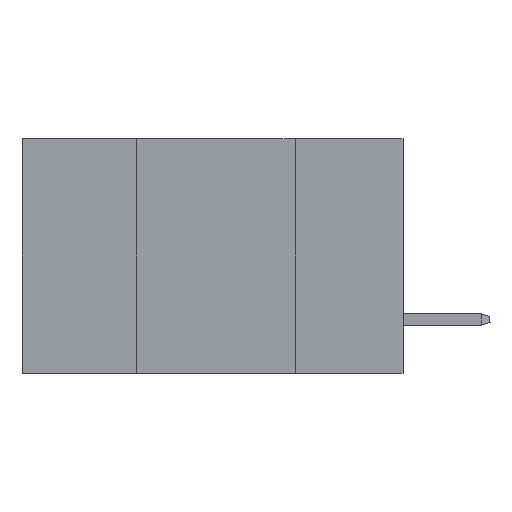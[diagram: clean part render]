
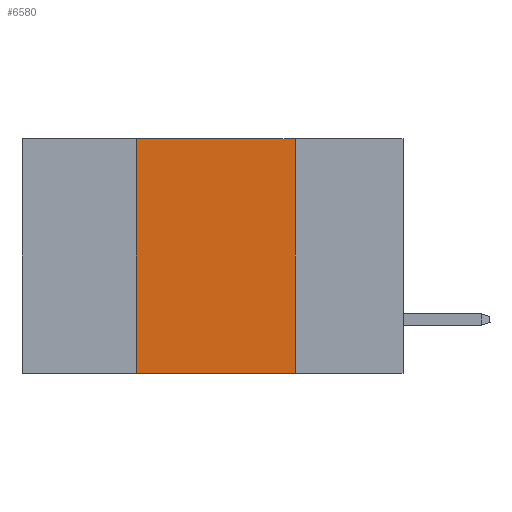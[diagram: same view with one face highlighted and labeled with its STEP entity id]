
A CAD part, left-side view. The second image highlights one B-rep face of the part: STEP entity #6580.
In plain terms, the highlighted planar face has unit normal (-1, 0, 0).
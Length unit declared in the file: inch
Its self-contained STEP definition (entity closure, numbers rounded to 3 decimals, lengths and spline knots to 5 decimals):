
#462 = ORIENTED_EDGE ( 'NONE', *, *, #1246, .F. ) ;
#648 = PLANE ( 'NONE',  #18231 ) ;
#1246 = EDGE_CURVE ( 'NONE', #4660, #2395, #1484, .T. ) ;
#1484 = LINE ( 'NONE', #4633, #2596 ) ;
#2219 = ORIENTED_EDGE ( 'NONE', *, *, #6779, .F. ) ;
#2395 = VERTEX_POINT ( 'NONE', #5164 ) ;
#2596 = VECTOR ( 'NONE', #7207, 39.37008 ) ;
#3591 = DIRECTION ( 'NONE',  ( 1., 0., 0. ) ) ;
#4169 = VERTEX_POINT ( 'NONE', #14268 ) ;
#4259 = DIRECTION ( 'NONE',  ( 0., 0., 1. ) ) ;
#4633 = CARTESIAN_POINT ( 'NONE',  ( 0., 0.6, 0. ) ) ;
#4660 = VERTEX_POINT ( 'NONE', #18342 ) ;
#5164 = CARTESIAN_POINT ( 'NONE',  ( 0., 0.17, 0. ) ) ;
#5970 = CARTESIAN_POINT ( 'NONE',  ( 0., 0.42, 0. ) ) ;
#6441 = CARTESIAN_POINT ( 'NONE',  ( 0., 0.6, 0. ) ) ;
#6580 = ADVANCED_FACE ( 'NONE', ( #13741 ), #648, .F. ) ;
#6779 = EDGE_CURVE ( 'NONE', #4169, #4660, #9993, .T. ) ;
#7207 = DIRECTION ( 'NONE',  ( 0., -1., 0. ) ) ;
#7555 = EDGE_LOOP ( 'NONE', ( #17619, #462, #2219, #8541 ) ) ;
#8541 = ORIENTED_EDGE ( 'NONE', *, *, #12636, .T. ) ;
#8994 = VERTEX_POINT ( 'NONE', #17352 ) ;
#9227 = DIRECTION ( 'NONE',  ( 0., 0., -1. ) ) ;
#9430 = DIRECTION ( 'NONE',  ( 0., 0., -1. ) ) ;
#9993 = LINE ( 'NONE', #5970, #18247 ) ;
#10327 = CARTESIAN_POINT ( 'NONE',  ( 0., 0.6, -0.37 ) ) ;
#10407 = EDGE_CURVE ( 'NONE', #2395, #8994, #10965, .T. ) ;
#10965 = LINE ( 'NONE', #18003, #18330 ) ;
#12636 = EDGE_CURVE ( 'NONE', #4169, #8994, #18630, .T. ) ;
#13528 = VECTOR ( 'NONE', #16126, 39.37008 ) ;
#13741 = FACE_OUTER_BOUND ( 'NONE', #7555, .T. ) ;
#14268 = CARTESIAN_POINT ( 'NONE',  ( 0., 0.42, -0.37 ) ) ;
#16126 = DIRECTION ( 'NONE',  ( 0., -1., 0. ) ) ;
#17352 = CARTESIAN_POINT ( 'NONE',  ( 0., 0.17, -0.37 ) ) ;
#17619 = ORIENTED_EDGE ( 'NONE', *, *, #10407, .F. ) ;
#18003 = CARTESIAN_POINT ( 'NONE',  ( 0., 0.17, 0. ) ) ;
#18231 = AXIS2_PLACEMENT_3D ( 'NONE', #6441, #3591, #9430 ) ;
#18247 = VECTOR ( 'NONE', #4259, 39.37008 ) ;
#18330 = VECTOR ( 'NONE', #9227, 39.37008 ) ;
#18342 = CARTESIAN_POINT ( 'NONE',  ( 0., 0.42, 0. ) ) ;
#18630 = LINE ( 'NONE', #10327, #13528 ) ;
